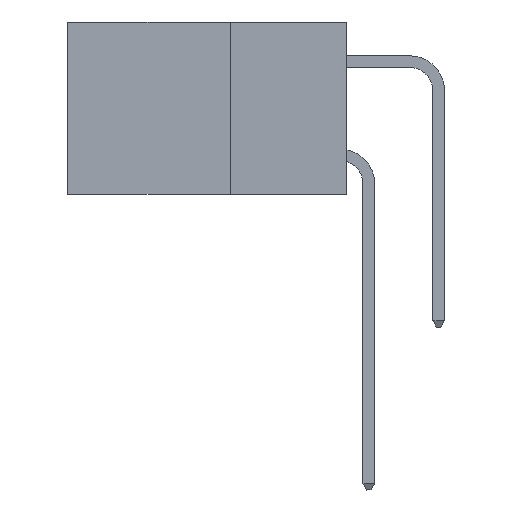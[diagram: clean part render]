
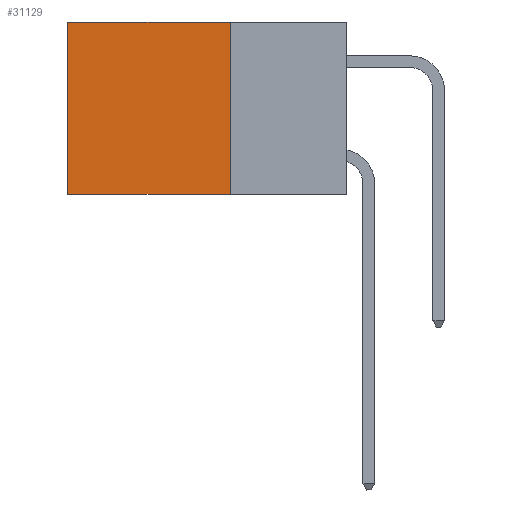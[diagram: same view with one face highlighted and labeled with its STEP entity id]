
A CAD part, left-side view. The second image highlights one B-rep face of the part: STEP entity #31129.
In plain terms, the highlighted planar face has unit normal (-1, 0, 0).
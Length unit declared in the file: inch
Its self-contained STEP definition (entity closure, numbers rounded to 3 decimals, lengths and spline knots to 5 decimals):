
#2758 = EDGE_CURVE ( 'NONE', #28903, #11291, #18071, .T. ) ;
#4164 = EDGE_LOOP ( 'NONE', ( #36849, #7497, #24263, #9429 ) ) ;
#7497 = ORIENTED_EDGE ( 'NONE', *, *, #26493, .F. ) ;
#7929 = CARTESIAN_POINT ( 'NONE',  ( 0.2875, 0.6, 0. ) ) ;
#8541 = VERTEX_POINT ( 'NONE', #26391 ) ;
#8971 = CARTESIAN_POINT ( 'NONE',  ( 0.2875, 0.25, 0. ) ) ;
#9429 = ORIENTED_EDGE ( 'NONE', *, *, #2758, .T. ) ;
#11291 = VERTEX_POINT ( 'NONE', #7929 ) ;
#13073 = CARTESIAN_POINT ( 'NONE',  ( 0.2875, 0.25, 0. ) ) ;
#13278 = DIRECTION ( 'NONE',  ( 0., 0., -1. ) ) ;
#13481 = FACE_OUTER_BOUND ( 'NONE', #4164, .T. ) ;
#14508 = CARTESIAN_POINT ( 'NONE',  ( 0.2875, 0.6, 0. ) ) ;
#15219 = DIRECTION ( 'NONE',  ( 0., 1., 0. ) ) ;
#16328 = DIRECTION ( 'NONE',  ( 1., 0., 0. ) ) ;
#16936 = VECTOR ( 'NONE', #15219, 39.37008 ) ;
#17726 = DIRECTION ( 'NONE',  ( 0., 1., 0. ) ) ;
#18071 = LINE ( 'NONE', #30509, #16936 ) ;
#18524 = DIRECTION ( 'NONE',  ( 0., 0., -1. ) ) ;
#19270 = VECTOR ( 'NONE', #17726, 39.37008 ) ;
#22004 = EDGE_CURVE ( 'NONE', #11291, #34862, #24676, .T. ) ;
#22245 = PLANE ( 'NONE',  #32488 ) ;
#24263 = ORIENTED_EDGE ( 'NONE', *, *, #26646, .F. ) ;
#24676 = LINE ( 'NONE', #14508, #39217 ) ;
#25801 = VECTOR ( 'NONE', #18524, 39.37008 ) ;
#26391 = CARTESIAN_POINT ( 'NONE',  ( 0.2875, 0.25, -0.37 ) ) ;
#26493 = EDGE_CURVE ( 'NONE', #8541, #34862, #32821, .T. ) ;
#26646 = EDGE_CURVE ( 'NONE', #28903, #8541, #30769, .T. ) ;
#28903 = VERTEX_POINT ( 'NONE', #35787 ) ;
#30509 = CARTESIAN_POINT ( 'NONE',  ( 0.2875, 0.25, 0. ) ) ;
#30769 = LINE ( 'NONE', #8971, #25801 ) ;
#31129 = ADVANCED_FACE ( 'NONE', ( #13481 ), #22245, .F. ) ;
#32488 = AXIS2_PLACEMENT_3D ( 'NONE', #13073, #16328, #13278 ) ;
#32621 = CARTESIAN_POINT ( 'NONE',  ( 0.2875, 0.25, -0.37 ) ) ;
#32821 = LINE ( 'NONE', #32621, #19270 ) ;
#33258 = DIRECTION ( 'NONE',  ( 0., 0., -1. ) ) ;
#34435 = CARTESIAN_POINT ( 'NONE',  ( 0.2875, 0.6, -0.37 ) ) ;
#34862 = VERTEX_POINT ( 'NONE', #34435 ) ;
#35787 = CARTESIAN_POINT ( 'NONE',  ( 0.2875, 0.25, 0. ) ) ;
#36849 = ORIENTED_EDGE ( 'NONE', *, *, #22004, .T. ) ;
#39217 = VECTOR ( 'NONE', #33258, 39.37008 ) ;
